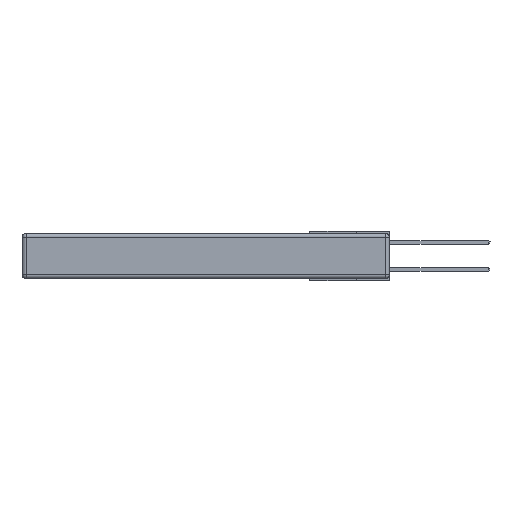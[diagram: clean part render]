
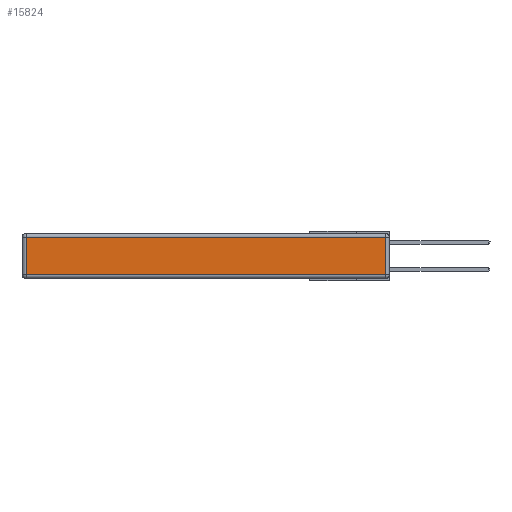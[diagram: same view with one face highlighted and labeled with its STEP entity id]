
A CAD part, left-side view. The second image highlights one B-rep face of the part: STEP entity #15824.
In plain terms, the highlighted planar face has unit normal (-1, 0, 0).
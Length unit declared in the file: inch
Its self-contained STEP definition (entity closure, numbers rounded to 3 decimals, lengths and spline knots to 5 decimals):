
#199 = EDGE_CURVE ( 'NONE', #6877, #10669, #22217, .T. ) ;
#504 = AXIS2_PLACEMENT_3D ( 'NONE', #3471, #8704, #21671 ) ;
#1734 = ORIENTED_EDGE ( 'NONE', *, *, #199, .T. ) ;
#3471 = CARTESIAN_POINT ( 'NONE',  ( 0., 0., -0.343 ) ) ;
#4308 = CARTESIAN_POINT ( 'NONE',  ( 0., 0.03, -0.343 ) ) ;
#5097 = EDGE_CURVE ( 'NONE', #10669, #32844, #12258, .T. ) ;
#5303 = FACE_OUTER_BOUND ( 'NONE', #6368, .T. ) ;
#5569 = DIRECTION ( 'NONE',  ( 0., 1., 0. ) ) ;
#5705 = EDGE_CURVE ( 'NONE', #32844, #11828, #26224, .T. ) ;
#6309 = ORIENTED_EDGE ( 'NONE', *, *, #14840, .T. ) ;
#6368 = EDGE_LOOP ( 'NONE', ( #10713, #12684, #6309, #1734 ) ) ;
#6877 = VERTEX_POINT ( 'NONE', #29368 ) ;
#8704 = DIRECTION ( 'NONE',  ( -1., 0., 0. ) ) ;
#8753 = CARTESIAN_POINT ( 'NONE',  ( 0., 0.03, -0.313 ) ) ;
#9247 = CARTESIAN_POINT ( 'NONE',  ( 0., 0.03, -0.03 ) ) ;
#10669 = VERTEX_POINT ( 'NONE', #33069 ) ;
#10713 = ORIENTED_EDGE ( 'NONE', *, *, #5097, .T. ) ;
#11828 = VERTEX_POINT ( 'NONE', #9247 ) ;
#12258 = LINE ( 'NONE', #17909, #19109 ) ;
#12684 = ORIENTED_EDGE ( 'NONE', *, *, #5705, .T. ) ;
#14677 = LINE ( 'NONE', #18236, #27590 ) ;
#14840 = EDGE_CURVE ( 'NONE', #11828, #6877, #14677, .T. ) ;
#15824 = ADVANCED_FACE ( 'NONE', ( #5303 ), #26751, .T. ) ;
#17909 = CARTESIAN_POINT ( 'NONE',  ( 0., 0., -0.313 ) ) ;
#18236 = CARTESIAN_POINT ( 'NONE',  ( 0., 2.75, -0.03 ) ) ;
#19109 = VECTOR ( 'NONE', #30754, 39.37008 ) ;
#19342 = VECTOR ( 'NONE', #22259, 39.37008 ) ;
#21671 = DIRECTION ( 'NONE',  ( 0., 0., 1. ) ) ;
#22217 = LINE ( 'NONE', #31797, #25500 ) ;
#22259 = DIRECTION ( 'NONE',  ( 0., 0., 1. ) ) ;
#25500 = VECTOR ( 'NONE', #29215, 39.37008 ) ;
#26224 = LINE ( 'NONE', #4308, #19342 ) ;
#26751 = PLANE ( 'NONE',  #504 ) ;
#27590 = VECTOR ( 'NONE', #5569, 39.37008 ) ;
#29215 = DIRECTION ( 'NONE',  ( 0., 0., -1. ) ) ;
#29368 = CARTESIAN_POINT ( 'NONE',  ( 0., 2.72, -0.03 ) ) ;
#30754 = DIRECTION ( 'NONE',  ( 0., -1., 0. ) ) ;
#31797 = CARTESIAN_POINT ( 'NONE',  ( 0., 2.72, -0.343 ) ) ;
#32844 = VERTEX_POINT ( 'NONE', #8753 ) ;
#33069 = CARTESIAN_POINT ( 'NONE',  ( 0., 2.72, -0.313 ) ) ;
